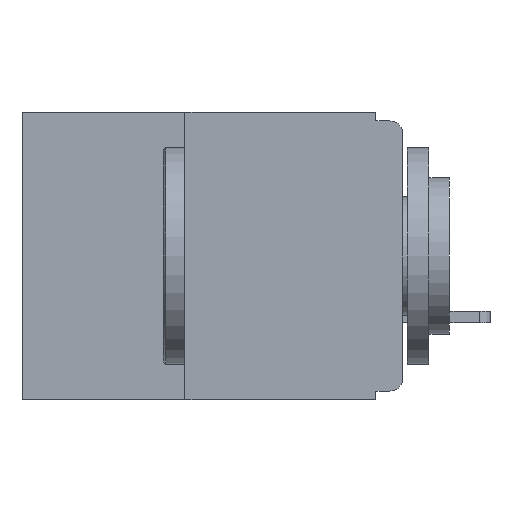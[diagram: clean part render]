
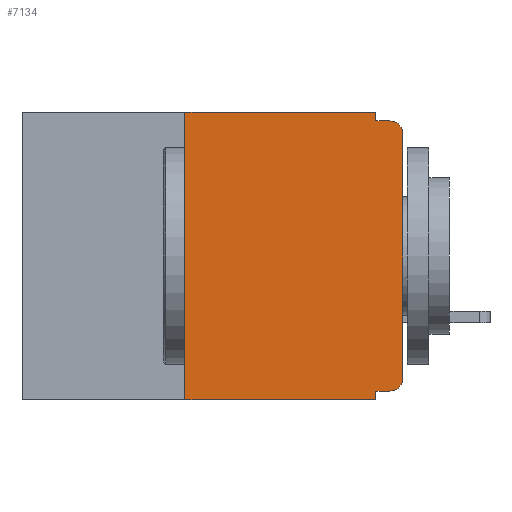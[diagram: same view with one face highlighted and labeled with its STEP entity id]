
A CAD part, left-side view. The second image highlights one B-rep face of the part: STEP entity #7134.
In plain terms, the highlighted planar face has unit normal (-1, 0, 0).
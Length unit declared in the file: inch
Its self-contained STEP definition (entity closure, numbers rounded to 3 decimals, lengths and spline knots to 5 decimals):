
#10 = ORIENTED_EDGE ( 'NONE', *, *, #13828, .T. ) ;
#132 = EDGE_LOOP ( 'NONE', ( #1438, #9080, #16097, #4719, #7025, #10253, #1219, #9673, #15692, #10 ) ) ;
#1219 = ORIENTED_EDGE ( 'NONE', *, *, #2592, .T. ) ;
#1261 = DIRECTION ( 'NONE',  ( 0., 0., -1. ) ) ;
#1337 = DIRECTION ( 'NONE',  ( 0., -1., 0. ) ) ;
#1394 = EDGE_CURVE ( 'NONE', #6095, #13093, #17431, .T. ) ;
#1438 = ORIENTED_EDGE ( 'NONE', *, *, #4724, .T. ) ;
#1634 = CARTESIAN_POINT ( 'NONE',  ( 0., 0.031, 0. ) ) ;
#1756 = CARTESIAN_POINT ( 'NONE',  ( 0., 0.031, 0. ) ) ;
#2592 = EDGE_CURVE ( 'NONE', #6974, #13093, #9785, .T. ) ;
#3980 = VERTEX_POINT ( 'NONE', #1756 ) ;
#4269 = VECTOR ( 'NONE', #19810, 39.37008 ) ;
#4289 = LINE ( 'NONE', #19970, #4269 ) ;
#4719 = ORIENTED_EDGE ( 'NONE', *, *, #10712, .F. ) ;
#4724 = EDGE_CURVE ( 'NONE', #7593, #7882, #5405, .T. ) ;
#4908 = CARTESIAN_POINT ( 'NONE',  ( 0., 0.031, -0.33 ) ) ;
#4974 = EDGE_CURVE ( 'NONE', #6974, #17065, #4289, .T. ) ;
#5311 = VECTOR ( 'NONE', #14743, 39.37008 ) ;
#5405 = LINE ( 'NONE', #14478, #5311 ) ;
#5459 = VERTEX_POINT ( 'NONE', #8392 ) ;
#5623 = DIRECTION ( 'NONE',  ( 0., 0., -1. ) ) ;
#6095 = VERTEX_POINT ( 'NONE', #15190 ) ;
#6781 = CARTESIAN_POINT ( 'NONE',  ( 0., 0.437, -0.33 ) ) ;
#6974 = VERTEX_POINT ( 'NONE', #7078 ) ;
#7025 = ORIENTED_EDGE ( 'NONE', *, *, #10170, .F. ) ;
#7078 = CARTESIAN_POINT ( 'NONE',  ( 0., 0.25, -0.33 ) ) ;
#7134 = ADVANCED_FACE ( 'NONE', ( #19911 ), #18808, .F. ) ;
#7504 = VECTOR ( 'NONE', #1261, 39.37008 ) ;
#7539 = CARTESIAN_POINT ( 'NONE',  ( 0., 0.031, -0.33 ) ) ;
#7593 = VERTEX_POINT ( 'NONE', #7782 ) ;
#7598 = LINE ( 'NONE', #1634, #7504 ) ;
#7782 = CARTESIAN_POINT ( 'NONE',  ( 0., 0., -0.305 ) ) ;
#7882 = VERTEX_POINT ( 'NONE', #17133 ) ;
#8037 = EDGE_CURVE ( 'NONE', #5459, #9060, #18610, .T. ) ;
#8392 = CARTESIAN_POINT ( 'NONE',  ( 0., 0.031, -0.01 ) ) ;
#9060 = VERTEX_POINT ( 'NONE', #11678 ) ;
#9080 = ORIENTED_EDGE ( 'NONE', *, *, #16412, .T. ) ;
#9673 = ORIENTED_EDGE ( 'NONE', *, *, #1394, .F. ) ;
#9785 = LINE ( 'NONE', #6781, #9801 ) ;
#9801 = VECTOR ( 'NONE', #1337, 39.37008 ) ;
#10019 = VECTOR ( 'NONE', #13518, 39.37008 ) ;
#10036 = DIRECTION ( 'NONE',  ( 0., 0., -1. ) ) ;
#10081 = DIRECTION ( 'NONE',  ( -1., 0., 0. ) ) ;
#10152 = CARTESIAN_POINT ( 'NONE',  ( 0., 0.015, -0.025 ) ) ;
#10170 = EDGE_CURVE ( 'NONE', #17065, #3980, #10363, .T. ) ;
#10248 = CIRCLE ( 'NONE', #19467, 0.015 ) ;
#10253 = ORIENTED_EDGE ( 'NONE', *, *, #4974, .F. ) ;
#10363 = LINE ( 'NONE', #13658, #10019 ) ;
#10483 = VECTOR ( 'NONE', #19259, 39.37008 ) ;
#10508 = LINE ( 'NONE', #19372, #10483 ) ;
#10712 = EDGE_CURVE ( 'NONE', #3980, #5459, #7598, .T. ) ;
#11233 = CARTESIAN_POINT ( 'NONE',  ( 0., 0.25, 0. ) ) ;
#11678 = CARTESIAN_POINT ( 'NONE',  ( 0., 0.015, -0.01 ) ) ;
#11909 = CARTESIAN_POINT ( 'NONE',  ( 0., 0.015, -0.32 ) ) ;
#12560 = VERTEX_POINT ( 'NONE', #11909 ) ;
#13093 = VERTEX_POINT ( 'NONE', #7539 ) ;
#13518 = DIRECTION ( 'NONE',  ( 0., -1., 0. ) ) ;
#13658 = CARTESIAN_POINT ( 'NONE',  ( 0., 0.437, 0. ) ) ;
#13828 = EDGE_CURVE ( 'NONE', #12560, #7593, #10248, .T. ) ;
#13869 = CIRCLE ( 'NONE', #14215, 0.015 ) ;
#14215 = AXIS2_PLACEMENT_3D ( 'NONE', #10152, #10081, #10036 ) ;
#14478 = CARTESIAN_POINT ( 'NONE',  ( 0., 0., 0. ) ) ;
#14743 = DIRECTION ( 'NONE',  ( 0., 0., 1. ) ) ;
#15190 = CARTESIAN_POINT ( 'NONE',  ( 0., 0.031, -0.32 ) ) ;
#15692 = ORIENTED_EDGE ( 'NONE', *, *, #17289, .F. ) ;
#16097 = ORIENTED_EDGE ( 'NONE', *, *, #8037, .F. ) ;
#16412 = EDGE_CURVE ( 'NONE', #7882, #9060, #13869, .T. ) ;
#16488 = VECTOR ( 'NONE', #5623, 39.37008 ) ;
#17065 = VERTEX_POINT ( 'NONE', #11233 ) ;
#17133 = CARTESIAN_POINT ( 'NONE',  ( 0., 0., -0.025 ) ) ;
#17257 = AXIS2_PLACEMENT_3D ( 'NONE', #19053, #18806, #18790 ) ;
#17289 = EDGE_CURVE ( 'NONE', #12560, #6095, #10508, .T. ) ;
#17431 = LINE ( 'NONE', #4908, #16488 ) ;
#18138 = VECTOR ( 'NONE', #20014, 39.37008 ) ;
#18610 = LINE ( 'NONE', #19794, #18138 ) ;
#18790 = DIRECTION ( 'NONE',  ( 0., 0., -1. ) ) ;
#18806 = DIRECTION ( 'NONE',  ( 1., 0., 0. ) ) ;
#18808 = PLANE ( 'NONE',  #17257 ) ;
#18977 = DIRECTION ( 'NONE',  ( 0., 0., -1. ) ) ;
#19025 = DIRECTION ( 'NONE',  ( -1., 0., 0. ) ) ;
#19053 = CARTESIAN_POINT ( 'NONE',  ( 0., 0.437, 0. ) ) ;
#19259 = DIRECTION ( 'NONE',  ( 0., 1., 0. ) ) ;
#19307 = CARTESIAN_POINT ( 'NONE',  ( 0., 0.015, -0.305 ) ) ;
#19372 = CARTESIAN_POINT ( 'NONE',  ( 0., 0., -0.32 ) ) ;
#19467 = AXIS2_PLACEMENT_3D ( 'NONE', #19307, #19025, #18977 ) ;
#19794 = CARTESIAN_POINT ( 'NONE',  ( 0., 0., -0.01 ) ) ;
#19810 = DIRECTION ( 'NONE',  ( 0., 0., 1. ) ) ;
#19911 = FACE_OUTER_BOUND ( 'NONE', #132, .T. ) ;
#19970 = CARTESIAN_POINT ( 'NONE',  ( 0., 0.25, -0.33 ) ) ;
#20014 = DIRECTION ( 'NONE',  ( 0., -1., 0. ) ) ;
